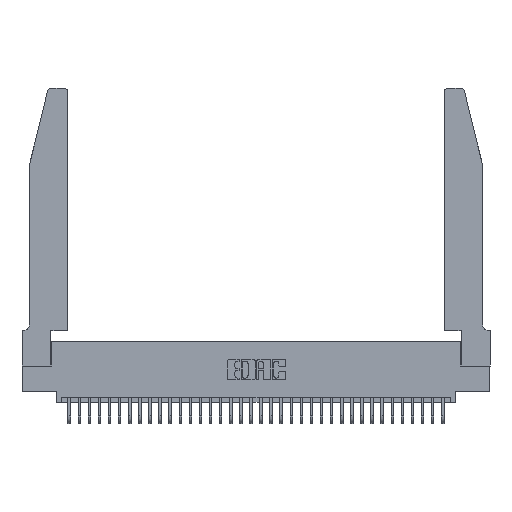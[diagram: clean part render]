
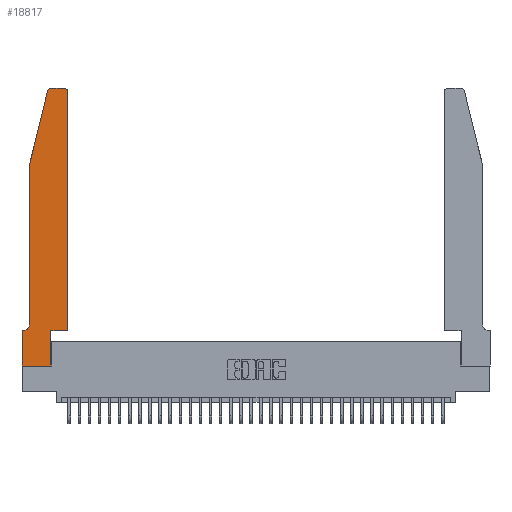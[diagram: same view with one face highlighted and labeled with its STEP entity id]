
A CAD part, top view. The second image highlights one B-rep face of the part: STEP entity #18817.
In plain terms, the highlighted planar face has unit normal (0, 0, 1).
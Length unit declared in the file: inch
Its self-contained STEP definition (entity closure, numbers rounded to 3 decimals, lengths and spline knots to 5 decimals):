
#116 = VERTEX_POINT ( 'NONE', #27991 ) ;
#186 = EDGE_CURVE ( 'NONE', #12566, #116, #27668, .T. ) ;
#253 = PLANE ( 'NONE',  #35304 ) ;
#483 = VERTEX_POINT ( 'NONE', #18062 ) ;
#1088 = ORIENTED_EDGE ( 'NONE', *, *, #2983, .T. ) ;
#1096 = LINE ( 'NONE', #19593, #30567 ) ;
#1302 = CIRCLE ( 'NONE', #32189, 0.03 ) ;
#2086 = VERTEX_POINT ( 'NONE', #28719 ) ;
#2088 = CARTESIAN_POINT ( 'NONE',  ( 0., 0., 0.37 ) ) ;
#2400 = ORIENTED_EDGE ( 'NONE', *, *, #21197, .T. ) ;
#2418 = EDGE_CURVE ( 'NONE', #34356, #2086, #12378, .T. ) ;
#2888 = CARTESIAN_POINT ( 'NONE',  ( 0.0755, 2., 0.37 ) ) ;
#2983 = EDGE_CURVE ( 'NONE', #35853, #35595, #1096, .T. ) ;
#3070 = ORIENTED_EDGE ( 'NONE', *, *, #186, .T. ) ;
#3181 = CARTESIAN_POINT ( 'NONE',  ( 0.4205, 2.75, 0.37 ) ) ;
#3189 = CARTESIAN_POINT ( 'NONE',  ( 0.2865, 0.35, 0.37 ) ) ;
#3450 = ORIENTED_EDGE ( 'NONE', *, *, #15764, .T. ) ;
#3575 = DIRECTION ( 'NONE',  ( 0., 0., 1. ) ) ;
#3590 = CARTESIAN_POINT ( 'NONE',  ( 0., 0.35, 0.37 ) ) ;
#4380 = EDGE_CURVE ( 'NONE', #18781, #483, #17215, .T. ) ;
#5126 = VERTEX_POINT ( 'NONE', #23683 ) ;
#5249 = DIRECTION ( 'NONE',  ( 0., 1., 0. ) ) ;
#5308 = VECTOR ( 'NONE', #8779, 39.37008 ) ;
#5367 = CARTESIAN_POINT ( 'NONE',  ( 0.2605, 2.75, 0.37 ) ) ;
#5567 = EDGE_LOOP ( 'NONE', ( #3070, #32768, #19032, #29256, #13903, #9360, #23828, #12940, #2400, #28636, #1088, #3450 ) ) ;
#5631 = VECTOR ( 'NONE', #22158, 39.37008 ) ;
#6573 = VERTEX_POINT ( 'NONE', #12554 ) ;
#7447 = LINE ( 'NONE', #22929, #21840 ) ;
#7699 = CARTESIAN_POINT ( 'NONE',  ( 0.25487, 2.72718, 0.37 ) ) ;
#8298 = CARTESIAN_POINT ( 'NONE',  ( 0.4505, 2.72, 0.37 ) ) ;
#8779 = DIRECTION ( 'NONE',  ( -0.239, -0.971, 0. ) ) ;
#9360 = ORIENTED_EDGE ( 'NONE', *, *, #20066, .T. ) ;
#10116 = VECTOR ( 'NONE', #35173, 39.37008 ) ;
#10666 = FACE_OUTER_BOUND ( 'NONE', #5567, .T. ) ;
#11133 = EDGE_CURVE ( 'NONE', #2086, #5126, #26817, .T. ) ;
#11345 = EDGE_CURVE ( 'NONE', #16089, #18781, #12950, .T. ) ;
#11805 = EDGE_CURVE ( 'NONE', #116, #16089, #36431, .T. ) ;
#11829 = DIRECTION ( 'NONE',  ( 0., 0., 1. ) ) ;
#12086 = DIRECTION ( 'NONE',  ( 0., -1., 0. ) ) ;
#12378 = LINE ( 'NONE', #2088, #5631 ) ;
#12554 = CARTESIAN_POINT ( 'NONE',  ( 0.2865, 0.35, 0.37 ) ) ;
#12566 = VERTEX_POINT ( 'NONE', #3181 ) ;
#12940 = ORIENTED_EDGE ( 'NONE', *, *, #11133, .T. ) ;
#12950 = LINE ( 'NONE', #2888, #5308 ) ;
#13903 = ORIENTED_EDGE ( 'NONE', *, *, #19565, .T. ) ;
#14438 = AXIS2_PLACEMENT_3D ( 'NONE', #16694, #36443, #19571 ) ;
#15380 = VECTOR ( 'NONE', #12086, 39.37008 ) ;
#15387 = CARTESIAN_POINT ( 'NONE',  ( 0.0755, 0.35, 0.37 ) ) ;
#15764 = EDGE_CURVE ( 'NONE', #35595, #12566, #1302, .T. ) ;
#15934 = CARTESIAN_POINT ( 'NONE',  ( 0.0055, 0.42, 0.37 ) ) ;
#15976 = LINE ( 'NONE', #15387, #10116 ) ;
#16089 = VERTEX_POINT ( 'NONE', #7699 ) ;
#16694 = CARTESIAN_POINT ( 'NONE',  ( 0.284, 2.72, 0.37 ) ) ;
#17215 = LINE ( 'NONE', #23476, #15380 ) ;
#18062 = CARTESIAN_POINT ( 'NONE',  ( 0.0755, 0.42, 0.37 ) ) ;
#18648 = LINE ( 'NONE', #3189, #32773 ) ;
#18781 = VERTEX_POINT ( 'NONE', #22982 ) ;
#18817 = ADVANCED_FACE ( 'NONE', ( #10666 ), #253, .T. ) ;
#18819 = DIRECTION ( 'NONE',  ( -1., 0., 0. ) ) ;
#19032 = ORIENTED_EDGE ( 'NONE', *, *, #11345, .T. ) ;
#19285 = VECTOR ( 'NONE', #19356, 39.37008 ) ;
#19356 = DIRECTION ( 'NONE',  ( 1., 0., 0. ) ) ;
#19565 = EDGE_CURVE ( 'NONE', #483, #34155, #32843, .T. ) ;
#19571 = DIRECTION ( 'NONE',  ( 1., 0., 0. ) ) ;
#19593 = CARTESIAN_POINT ( 'NONE',  ( 0.4505, 0.35, 0.37 ) ) ;
#20066 = EDGE_CURVE ( 'NONE', #34155, #34356, #15976, .T. ) ;
#20158 = VECTOR ( 'NONE', #31044, 39.37008 ) ;
#20798 = CARTESIAN_POINT ( 'NONE',  ( 0.4205, 2.72, 0.37 ) ) ;
#21197 = EDGE_CURVE ( 'NONE', #5126, #6573, #18648, .T. ) ;
#21840 = VECTOR ( 'NONE', #31409, 39.37008 ) ;
#22158 = DIRECTION ( 'NONE',  ( 0., -1., 0. ) ) ;
#22929 = CARTESIAN_POINT ( 'NONE',  ( 0.4505, 0.35, 0.37 ) ) ;
#22982 = CARTESIAN_POINT ( 'NONE',  ( 0.0755, 2., 0.37 ) ) ;
#23476 = CARTESIAN_POINT ( 'NONE',  ( 0.0755, 2., 0.37 ) ) ;
#23656 = DIRECTION ( 'NONE',  ( 1., 0., 0. ) ) ;
#23683 = CARTESIAN_POINT ( 'NONE',  ( 0.2865, 0., 0.37 ) ) ;
#23828 = ORIENTED_EDGE ( 'NONE', *, *, #2418, .T. ) ;
#23837 = CARTESIAN_POINT ( 'NONE',  ( 0.4505, 0.35, 0.37 ) ) ;
#26817 = LINE ( 'NONE', #30591, #19285 ) ;
#27668 = LINE ( 'NONE', #5367, #20158 ) ;
#27991 = CARTESIAN_POINT ( 'NONE',  ( 0.284, 2.75, 0.37 ) ) ;
#28636 = ORIENTED_EDGE ( 'NONE', *, *, #30938, .T. ) ;
#28719 = CARTESIAN_POINT ( 'NONE',  ( 0., 0., 0.37 ) ) ;
#28892 = CARTESIAN_POINT ( 'NONE',  ( 0., 0.35, 0.37 ) ) ;
#29256 = ORIENTED_EDGE ( 'NONE', *, *, #4380, .T. ) ;
#30567 = VECTOR ( 'NONE', #5249, 39.37008 ) ;
#30591 = CARTESIAN_POINT ( 'NONE',  ( 0., 0., 0.37 ) ) ;
#30938 = EDGE_CURVE ( 'NONE', #6573, #35853, #7447, .T. ) ;
#31044 = DIRECTION ( 'NONE',  ( -1., 0., 0. ) ) ;
#31170 = CARTESIAN_POINT ( 'NONE',  ( 0.0055, 0.35, 0.37 ) ) ;
#31409 = DIRECTION ( 'NONE',  ( 1., 0., 0. ) ) ;
#31625 = DIRECTION ( 'NONE',  ( 0., 1., 0. ) ) ;
#31711 = DIRECTION ( 'NONE',  ( 1., 0., 0. ) ) ;
#32189 = AXIS2_PLACEMENT_3D ( 'NONE', #20798, #3575, #23656 ) ;
#32768 = ORIENTED_EDGE ( 'NONE', *, *, #11805, .T. ) ;
#32773 = VECTOR ( 'NONE', #31625, 39.37008 ) ;
#32843 = CIRCLE ( 'NONE', #35785, 0.07 ) ;
#34155 = VERTEX_POINT ( 'NONE', #31170 ) ;
#34356 = VERTEX_POINT ( 'NONE', #3590 ) ;
#35173 = DIRECTION ( 'NONE',  ( -1., 0., 0. ) ) ;
#35304 = AXIS2_PLACEMENT_3D ( 'NONE', #28892, #11829, #31711 ) ;
#35595 = VERTEX_POINT ( 'NONE', #8298 ) ;
#35706 = DIRECTION ( 'NONE',  ( 0., 0., -1. ) ) ;
#35785 = AXIS2_PLACEMENT_3D ( 'NONE', #15934, #35706, #18819 ) ;
#35853 = VERTEX_POINT ( 'NONE', #23837 ) ;
#36431 = CIRCLE ( 'NONE', #14438, 0.03 ) ;
#36443 = DIRECTION ( 'NONE',  ( 0., 0., 1. ) ) ;
